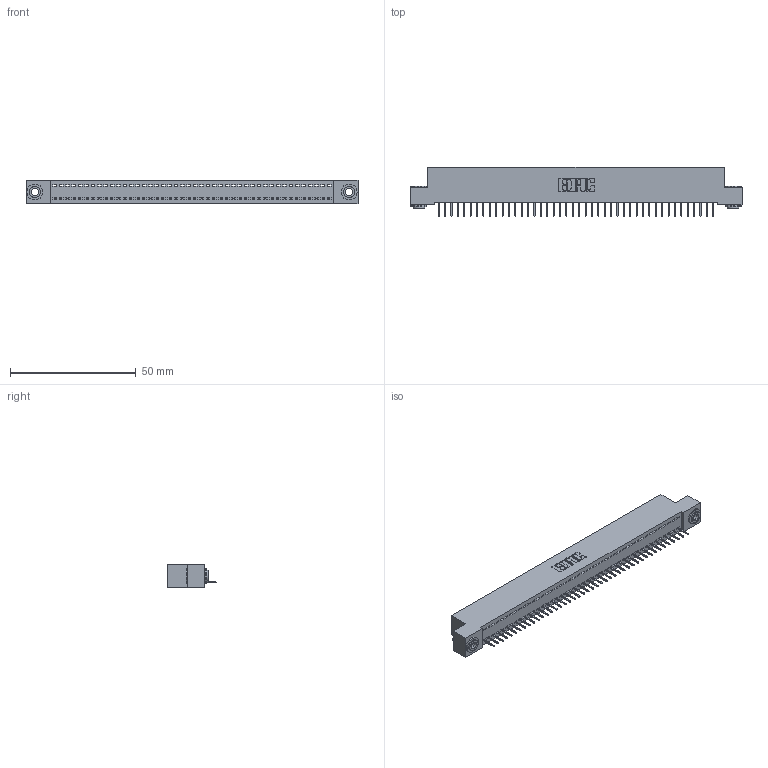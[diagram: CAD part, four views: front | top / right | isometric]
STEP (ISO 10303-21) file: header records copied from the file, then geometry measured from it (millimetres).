
FILE_DESCRIPTION (( 'STEP AP203' ), '1' );
FILE_NAME ('392-044-524-103.STEP', '2018-08-16T14:59:06', ( '' ), ( '' ), 'SwSTEP 2.0', 'SolidWorks 2016', '' );
FILE_SCHEMA (( 'CONFIG_CONTROL_DESIGN' ));
Length unit declared in the file: inch
Products named in the file (4): 342 Part_.156 TH; 345-292-001_345-293-124; 342-250-002_345-250-002-102; 392-044-524-103
Assembly tree (47 placements, depth 2):
  392-044-524-103
    342 Part_.156 TH
    345-292-001_345-293-124  x44
    342-250-002_345-250-002-102  x2
Bounding box: 132.08 x 19.69 x 9.4 mm (x, y, z)
Volume: 11437.2 mm3; surface area: 16518.6 mm2
Topology: 47 solids, 47 shells, 2876 faces, 8295 edges, 5350 vertices
Faces by surface type: plane 2188, cylinder 680, cone 8
Entity records: 27232 total; most frequent: CARTESIAN_POINT 4673, ORIENTED_EDGE 4646, DIRECTION 3973, EDGE_CURVE 2323, VECTOR 2175, LINE 2175, VERTEX_POINT 1542, AXIS2_PLACEMENT_3D 899
